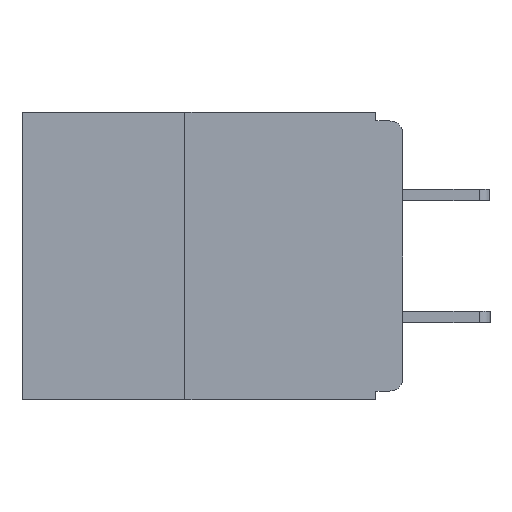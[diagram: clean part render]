
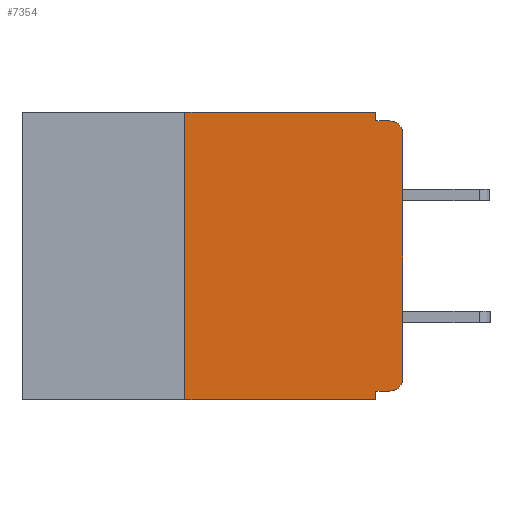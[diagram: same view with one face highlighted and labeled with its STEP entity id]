
A CAD part, left-side view. The second image highlights one B-rep face of the part: STEP entity #7354.
In plain terms, the highlighted planar face has unit normal (-1, 0, 0).
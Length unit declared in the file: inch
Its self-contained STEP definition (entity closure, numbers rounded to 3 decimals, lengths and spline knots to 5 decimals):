
#129 = CARTESIAN_POINT ( 'NONE',  ( 0., 0.031, 0. ) ) ;
#179 = VECTOR ( 'NONE', #5803, 39.37008 ) ;
#460 = VECTOR ( 'NONE', #25279, 39.37008 ) ;
#945 = LINE ( 'NONE', #12245, #12356 ) ;
#1184 = LINE ( 'NONE', #13967, #460 ) ;
#1272 = VERTEX_POINT ( 'NONE', #20236 ) ;
#1957 = CARTESIAN_POINT ( 'NONE',  ( 0., 0.031, 0. ) ) ;
#2381 = VECTOR ( 'NONE', #25674, 39.37008 ) ;
#2645 = CARTESIAN_POINT ( 'NONE',  ( 0., 0.437, 0. ) ) ;
#2837 = VERTEX_POINT ( 'NONE', #18584 ) ;
#3210 = CARTESIAN_POINT ( 'NONE',  ( 0., 0., -0.305 ) ) ;
#3548 = EDGE_CURVE ( 'NONE', #29039, #5648, #14529, .T. ) ;
#3607 = EDGE_CURVE ( 'NONE', #1272, #5648, #945, .T. ) ;
#3826 = ORIENTED_EDGE ( 'NONE', *, *, #20519, .F. ) ;
#4038 = CARTESIAN_POINT ( 'NONE',  ( 0., 0.015, -0.025 ) ) ;
#4434 = VERTEX_POINT ( 'NONE', #26495 ) ;
#5173 = VERTEX_POINT ( 'NONE', #15429 ) ;
#5290 = ORIENTED_EDGE ( 'NONE', *, *, #3607, .F. ) ;
#5308 = CARTESIAN_POINT ( 'NONE',  ( 0., 0.437, 0. ) ) ;
#5648 = VERTEX_POINT ( 'NONE', #14772 ) ;
#5803 = DIRECTION ( 'NONE',  ( 0., 1., 0. ) ) ;
#6030 = EDGE_CURVE ( 'NONE', #29039, #4434, #9788, .T. ) ;
#6333 = ORIENTED_EDGE ( 'NONE', *, *, #18662, .T. ) ;
#6359 = DIRECTION ( 'NONE',  ( 0., 0., -1. ) ) ;
#7354 = ADVANCED_FACE ( 'NONE', ( #27044 ), #23389, .F. ) ;
#8452 = VERTEX_POINT ( 'NONE', #129 ) ;
#8751 = DIRECTION ( 'NONE',  ( 0., 0., -1. ) ) ;
#9076 = VECTOR ( 'NONE', #27305, 39.37008 ) ;
#9174 = CARTESIAN_POINT ( 'NONE',  ( 0., 0.25, -0.33 ) ) ;
#9294 = VERTEX_POINT ( 'NONE', #3210 ) ;
#9382 = VERTEX_POINT ( 'NONE', #12682 ) ;
#9788 = LINE ( 'NONE', #9174, #9076 ) ;
#9799 = CARTESIAN_POINT ( 'NONE',  ( 0., 0., 0. ) ) ;
#9898 = DIRECTION ( 'NONE',  ( 0., 0., -1. ) ) ;
#10320 = AXIS2_PLACEMENT_3D ( 'NONE', #4038, #19978, #6359 ) ;
#12102 = CARTESIAN_POINT ( 'NONE',  ( 0., 0.015, -0.305 ) ) ;
#12245 = CARTESIAN_POINT ( 'NONE',  ( 0., 0.031, -0.33 ) ) ;
#12356 = VECTOR ( 'NONE', #25862, 39.37008 ) ;
#12682 = CARTESIAN_POINT ( 'NONE',  ( 0., 0., -0.025 ) ) ;
#13792 = CIRCLE ( 'NONE', #20125, 0.015 ) ;
#13967 = CARTESIAN_POINT ( 'NONE',  ( 0., 0., -0.01 ) ) ;
#14096 = EDGE_CURVE ( 'NONE', #9382, #5173, #27986, .T. ) ;
#14412 = DIRECTION ( 'NONE',  ( 0., 0., -1. ) ) ;
#14529 = LINE ( 'NONE', #18845, #2381 ) ;
#14772 = CARTESIAN_POINT ( 'NONE',  ( 0., 0.031, -0.33 ) ) ;
#14920 = ORIENTED_EDGE ( 'NONE', *, *, #22971, .F. ) ;
#14991 = VECTOR ( 'NONE', #8751, 39.37008 ) ;
#15130 = CARTESIAN_POINT ( 'NONE',  ( 0., 0.015, -0.32 ) ) ;
#15157 = EDGE_LOOP ( 'NONE', ( #6333, #27271, #3826, #29314, #14920, #22328, #17770, #5290, #17421, #18844 ) ) ;
#15429 = CARTESIAN_POINT ( 'NONE',  ( 0., 0.015, -0.01 ) ) ;
#15618 = LINE ( 'NONE', #21666, #179 ) ;
#16691 = DIRECTION ( 'NONE',  ( 0., 0., 1. ) ) ;
#17421 = ORIENTED_EDGE ( 'NONE', *, *, #28034, .F. ) ;
#17453 = CARTESIAN_POINT ( 'NONE',  ( 0., 0.25, -0.33 ) ) ;
#17770 = ORIENTED_EDGE ( 'NONE', *, *, #3548, .T. ) ;
#18264 = VERTEX_POINT ( 'NONE', #15130 ) ;
#18584 = CARTESIAN_POINT ( 'NONE',  ( 0., 0.031, -0.01 ) ) ;
#18662 = EDGE_CURVE ( 'NONE', #9294, #9382, #29092, .T. ) ;
#18844 = ORIENTED_EDGE ( 'NONE', *, *, #27258, .T. ) ;
#18845 = CARTESIAN_POINT ( 'NONE',  ( 0., 0.437, -0.33 ) ) ;
#18884 = LINE ( 'NONE', #2645, #29375 ) ;
#19978 = DIRECTION ( 'NONE',  ( -1., 0., 0. ) ) ;
#20125 = AXIS2_PLACEMENT_3D ( 'NONE', #12102, #27952, #14412 ) ;
#20236 = CARTESIAN_POINT ( 'NONE',  ( 0., 0.031, -0.32 ) ) ;
#20292 = LINE ( 'NONE', #1957, #14991 ) ;
#20519 = EDGE_CURVE ( 'NONE', #2837, #5173, #1184, .T. ) ;
#20849 = DIRECTION ( 'NONE',  ( 0., -1., 0. ) ) ;
#21666 = CARTESIAN_POINT ( 'NONE',  ( 0., 0., -0.32 ) ) ;
#22328 = ORIENTED_EDGE ( 'NONE', *, *, #6030, .F. ) ;
#22790 = AXIS2_PLACEMENT_3D ( 'NONE', #5308, #23481, #9898 ) ;
#22884 = EDGE_CURVE ( 'NONE', #8452, #2837, #20292, .T. ) ;
#22971 = EDGE_CURVE ( 'NONE', #4434, #8452, #18884, .T. ) ;
#23162 = VECTOR ( 'NONE', #16691, 39.37008 ) ;
#23389 = PLANE ( 'NONE',  #22790 ) ;
#23481 = DIRECTION ( 'NONE',  ( 1., 0., 0. ) ) ;
#25279 = DIRECTION ( 'NONE',  ( 0., -1., 0. ) ) ;
#25674 = DIRECTION ( 'NONE',  ( 0., -1., 0. ) ) ;
#25862 = DIRECTION ( 'NONE',  ( 0., 0., -1. ) ) ;
#26495 = CARTESIAN_POINT ( 'NONE',  ( 0., 0.25, 0. ) ) ;
#27044 = FACE_OUTER_BOUND ( 'NONE', #15157, .T. ) ;
#27258 = EDGE_CURVE ( 'NONE', #18264, #9294, #13792, .T. ) ;
#27271 = ORIENTED_EDGE ( 'NONE', *, *, #14096, .T. ) ;
#27305 = DIRECTION ( 'NONE',  ( 0., 0., 1. ) ) ;
#27952 = DIRECTION ( 'NONE',  ( -1., 0., 0. ) ) ;
#27986 = CIRCLE ( 'NONE', #10320, 0.015 ) ;
#28034 = EDGE_CURVE ( 'NONE', #18264, #1272, #15618, .T. ) ;
#29039 = VERTEX_POINT ( 'NONE', #17453 ) ;
#29092 = LINE ( 'NONE', #9799, #23162 ) ;
#29314 = ORIENTED_EDGE ( 'NONE', *, *, #22884, .F. ) ;
#29375 = VECTOR ( 'NONE', #20849, 39.37008 ) ;
